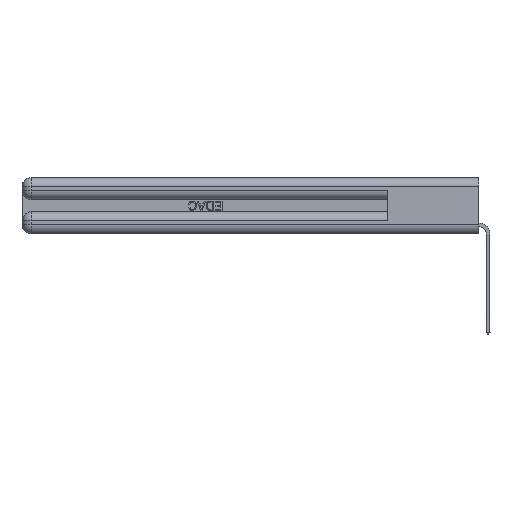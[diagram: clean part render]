
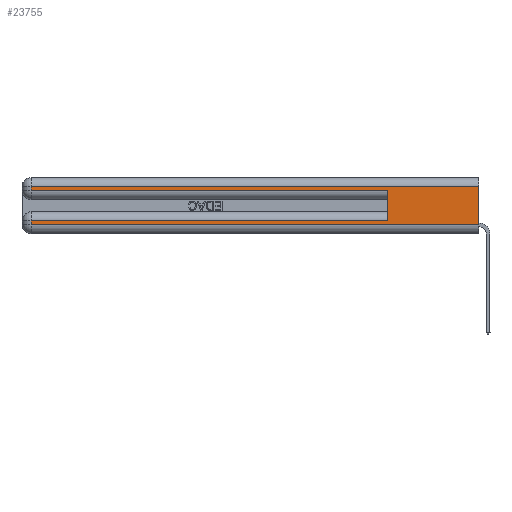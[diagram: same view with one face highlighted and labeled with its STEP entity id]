
A CAD part, left-side view. The second image highlights one B-rep face of the part: STEP entity #23755.
In plain terms, the highlighted planar face has unit normal (-1, 0, 0).
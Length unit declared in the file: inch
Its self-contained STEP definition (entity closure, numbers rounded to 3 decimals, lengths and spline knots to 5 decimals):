
#711 = EDGE_CURVE ( 'NONE', #16599, #3824, #28446, .T. ) ;
#792 = EDGE_LOOP ( 'NONE', ( #29269, #20768, #10871, #4319, #15294, #4552, #21554, #21903 ) ) ;
#2103 = VERTEX_POINT ( 'NONE', #3475 ) ;
#2161 = DIRECTION ( 'NONE',  ( 0., 0., -1. ) ) ;
#2744 = VERTEX_POINT ( 'NONE', #21832 ) ;
#3475 = CARTESIAN_POINT ( 'NONE',  ( 0., 2.94, 0.06 ) ) ;
#3777 = EDGE_CURVE ( 'NONE', #23959, #16599, #10199, .T. ) ;
#3824 = VERTEX_POINT ( 'NONE', #28449 ) ;
#4319 = ORIENTED_EDGE ( 'NONE', *, *, #25513, .T. ) ;
#4369 = VECTOR ( 'NONE', #31387, 39.37008 ) ;
#4552 = ORIENTED_EDGE ( 'NONE', *, *, #19758, .T. ) ;
#4864 = DIRECTION ( 'NONE',  ( 0., -1., 0. ) ) ;
#5454 = CARTESIAN_POINT ( 'NONE',  ( 0., 0.6, 0.285 ) ) ;
#6086 = CARTESIAN_POINT ( 'NONE',  ( 0., 2.94, 0.37 ) ) ;
#6854 = LINE ( 'NONE', #16805, #22440 ) ;
#7031 = LINE ( 'NONE', #16980, #19929 ) ;
#7295 = VECTOR ( 'NONE', #29210, 39.37008 ) ;
#7311 = CARTESIAN_POINT ( 'NONE',  ( 0., 0., 0.285 ) ) ;
#7338 = DIRECTION ( 'NONE',  ( 0., 0., -1. ) ) ;
#8880 = CARTESIAN_POINT ( 'NONE',  ( 0., 2.94, 0.31 ) ) ;
#9697 = EDGE_CURVE ( 'NONE', #26524, #10988, #22155, .T. ) ;
#9793 = PLANE ( 'NONE',  #17754 ) ;
#10199 = LINE ( 'NONE', #22405, #24216 ) ;
#10871 = ORIENTED_EDGE ( 'NONE', *, *, #711, .T. ) ;
#10988 = VERTEX_POINT ( 'NONE', #5454 ) ;
#11352 = DIRECTION ( 'NONE',  ( 0., 1., 0. ) ) ;
#11606 = DIRECTION ( 'NONE',  ( 0., 0., -1. ) ) ;
#11675 = LINE ( 'NONE', #28950, #16580 ) ;
#12904 = EDGE_CURVE ( 'NONE', #23959, #2744, #7031, .T. ) ;
#13485 = CARTESIAN_POINT ( 'NONE',  ( 0., 0.6, 0.085 ) ) ;
#15294 = ORIENTED_EDGE ( 'NONE', *, *, #9697, .F. ) ;
#16580 = VECTOR ( 'NONE', #11352, 39.37008 ) ;
#16599 = VERTEX_POINT ( 'NONE', #8880 ) ;
#16805 = CARTESIAN_POINT ( 'NONE',  ( 0., 2.94, 0.37 ) ) ;
#16980 = CARTESIAN_POINT ( 'NONE',  ( 0., 0., 0.37 ) ) ;
#17405 = EDGE_CURVE ( 'NONE', #2103, #2744, #24087, .T. ) ;
#17754 = AXIS2_PLACEMENT_3D ( 'NONE', #19722, #29700, #7338 ) ;
#18376 = VECTOR ( 'NONE', #4864, 39.37008 ) ;
#19722 = CARTESIAN_POINT ( 'NONE',  ( 0., 0., 0.37 ) ) ;
#19758 = EDGE_CURVE ( 'NONE', #26524, #21733, #11675, .T. ) ;
#19929 = VECTOR ( 'NONE', #2161, 39.37008 ) ;
#20104 = DIRECTION ( 'NONE',  ( 0., 1., 0. ) ) ;
#20768 = ORIENTED_EDGE ( 'NONE', *, *, #3777, .T. ) ;
#21554 = ORIENTED_EDGE ( 'NONE', *, *, #22407, .T. ) ;
#21733 = VERTEX_POINT ( 'NONE', #30880 ) ;
#21832 = CARTESIAN_POINT ( 'NONE',  ( 0., 0., 0.06 ) ) ;
#21903 = ORIENTED_EDGE ( 'NONE', *, *, #17405, .T. ) ;
#22155 = LINE ( 'NONE', #32159, #7295 ) ;
#22405 = CARTESIAN_POINT ( 'NONE',  ( 0., 0., 0.31 ) ) ;
#22407 = EDGE_CURVE ( 'NONE', #21733, #2103, #6854, .T. ) ;
#22440 = VECTOR ( 'NONE', #11606, 39.37008 ) ;
#23749 = CARTESIAN_POINT ( 'NONE',  ( 0., 0., 0.06 ) ) ;
#23755 = ADVANCED_FACE ( 'NONE', ( #32162 ), #9793, .F. ) ;
#23959 = VERTEX_POINT ( 'NONE', #26897 ) ;
#24087 = LINE ( 'NONE', #23749, #27074 ) ;
#24216 = VECTOR ( 'NONE', #20104, 39.37008 ) ;
#25513 = EDGE_CURVE ( 'NONE', #3824, #10988, #29669, .T. ) ;
#26524 = VERTEX_POINT ( 'NONE', #13485 ) ;
#26897 = CARTESIAN_POINT ( 'NONE',  ( 0., 0., 0.31 ) ) ;
#27074 = VECTOR ( 'NONE', #28664, 39.37008 ) ;
#28446 = LINE ( 'NONE', #6086, #4369 ) ;
#28449 = CARTESIAN_POINT ( 'NONE',  ( 0., 2.94, 0.285 ) ) ;
#28664 = DIRECTION ( 'NONE',  ( 0., -1., 0. ) ) ;
#28950 = CARTESIAN_POINT ( 'NONE',  ( 0., 0., 0.085 ) ) ;
#29210 = DIRECTION ( 'NONE',  ( 0., 0., 1. ) ) ;
#29269 = ORIENTED_EDGE ( 'NONE', *, *, #12904, .F. ) ;
#29669 = LINE ( 'NONE', #7311, #18376 ) ;
#29700 = DIRECTION ( 'NONE',  ( 1., 0., 0. ) ) ;
#30880 = CARTESIAN_POINT ( 'NONE',  ( 0., 2.94, 0.085 ) ) ;
#31387 = DIRECTION ( 'NONE',  ( 0., 0., -1. ) ) ;
#32159 = CARTESIAN_POINT ( 'NONE',  ( 0., 0.6, 0.145 ) ) ;
#32162 = FACE_OUTER_BOUND ( 'NONE', #792, .T. ) ;
